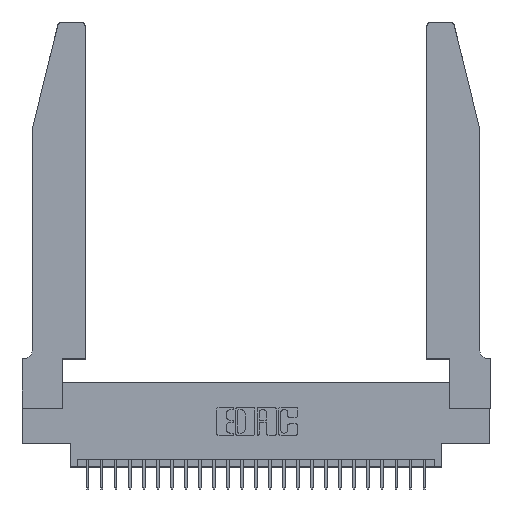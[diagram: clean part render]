
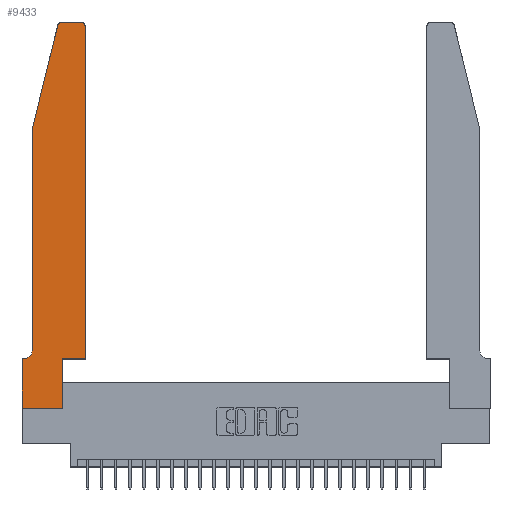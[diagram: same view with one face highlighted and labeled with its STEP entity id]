
A CAD part, top view. The second image highlights one B-rep face of the part: STEP entity #9433.
In plain terms, the highlighted planar face has unit normal (0, 0, 1).
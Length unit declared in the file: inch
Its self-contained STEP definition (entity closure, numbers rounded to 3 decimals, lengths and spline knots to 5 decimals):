
#201 = DIRECTION ( 'NONE',  ( 0., 0., 1. ) ) ;
#255 = CARTESIAN_POINT ( 'NONE',  ( 0.25487, 2.72718, 0.37 ) ) ;
#428 = EDGE_CURVE ( 'NONE', #19075, #12175, #15630, .T. ) ;
#579 = AXIS2_PLACEMENT_3D ( 'NONE', #21313, #201, #15273 ) ;
#582 = CARTESIAN_POINT ( 'NONE',  ( 0.4505, 0.35, 0.37 ) ) ;
#599 = DIRECTION ( 'NONE',  ( 0., -1., 0. ) ) ;
#766 = VERTEX_POINT ( 'NONE', #12396 ) ;
#1272 = CARTESIAN_POINT ( 'NONE',  ( 0.2865, 0.35, 0.37 ) ) ;
#1925 = VECTOR ( 'NONE', #23389, 39.37008 ) ;
#2009 = VERTEX_POINT ( 'NONE', #18621 ) ;
#2076 = VERTEX_POINT ( 'NONE', #255 ) ;
#2501 = VECTOR ( 'NONE', #21606, 39.37008 ) ;
#2733 = DIRECTION ( 'NONE',  ( -1., 0., 0. ) ) ;
#2997 = FACE_OUTER_BOUND ( 'NONE', #4580, .T. ) ;
#3164 = LINE ( 'NONE', #19623, #16791 ) ;
#3190 = CARTESIAN_POINT ( 'NONE',  ( 0.4505, 0.35, 0.37 ) ) ;
#3637 = DIRECTION ( 'NONE',  ( 1., 0., 0. ) ) ;
#3979 = ORIENTED_EDGE ( 'NONE', *, *, #20023, .T. ) ;
#4580 = EDGE_LOOP ( 'NONE', ( #16132, #8854, #22456, #3979, #19165, #18910, #22630, #10959, #16016, #23690, #14038, #8285 ) ) ;
#4980 = CARTESIAN_POINT ( 'NONE',  ( 0.0055, 0.42, 0.37 ) ) ;
#5750 = CARTESIAN_POINT ( 'NONE',  ( 0., 0.35, 0.37 ) ) ;
#5932 = CARTESIAN_POINT ( 'NONE',  ( 0.0755, 2., 0.37 ) ) ;
#6069 = LINE ( 'NONE', #582, #2501 ) ;
#7103 = CIRCLE ( 'NONE', #16468, 0.07 ) ;
#7587 = CARTESIAN_POINT ( 'NONE',  ( 0.4505, 2.72, 0.37 ) ) ;
#7709 = VECTOR ( 'NONE', #3637, 39.37008 ) ;
#7815 = VERTEX_POINT ( 'NONE', #7587 ) ;
#7955 = CARTESIAN_POINT ( 'NONE',  ( 0.2865, 0.35, 0.37 ) ) ;
#8285 = ORIENTED_EDGE ( 'NONE', *, *, #20357, .T. ) ;
#8297 = EDGE_CURVE ( 'NONE', #24174, #2009, #24781, .T. ) ;
#8361 = CARTESIAN_POINT ( 'NONE',  ( 0., 0., 0.37 ) ) ;
#8854 = ORIENTED_EDGE ( 'NONE', *, *, #17176, .T. ) ;
#9367 = LINE ( 'NONE', #20008, #7709 ) ;
#9433 = ADVANCED_FACE ( 'NONE', ( #2997 ), #18389, .T. ) ;
#9631 = CIRCLE ( 'NONE', #579, 0.03 ) ;
#10236 = CARTESIAN_POINT ( 'NONE',  ( 0.0755, 0.35, 0.37 ) ) ;
#10495 = CARTESIAN_POINT ( 'NONE',  ( 0.0055, 0.35, 0.37 ) ) ;
#10843 = EDGE_CURVE ( 'NONE', #15918, #26192, #7103, .T. ) ;
#10959 = ORIENTED_EDGE ( 'NONE', *, *, #19573, .T. ) ;
#11268 = DIRECTION ( 'NONE',  ( -1., 0., 0. ) ) ;
#11273 = EDGE_CURVE ( 'NONE', #26192, #24174, #24287, .T. ) ;
#11749 = VECTOR ( 'NONE', #21654, 39.37008 ) ;
#12175 = VERTEX_POINT ( 'NONE', #7955 ) ;
#12194 = LINE ( 'NONE', #5932, #21208 ) ;
#12396 = CARTESIAN_POINT ( 'NONE',  ( 0.0755, 2., 0.37 ) ) ;
#12456 = AXIS2_PLACEMENT_3D ( 'NONE', #5750, #15930, #24153 ) ;
#12502 = CARTESIAN_POINT ( 'NONE',  ( 0.284, 2.72, 0.37 ) ) ;
#13278 = CARTESIAN_POINT ( 'NONE',  ( 0.2605, 2.75, 0.37 ) ) ;
#13527 = CARTESIAN_POINT ( 'NONE',  ( 0.0755, 0.42, 0.37 ) ) ;
#14038 = ORIENTED_EDGE ( 'NONE', *, *, #14131, .T. ) ;
#14131 = EDGE_CURVE ( 'NONE', #22532, #7815, #17424, .T. ) ;
#15023 = EDGE_CURVE ( 'NONE', #2076, #766, #12194, .T. ) ;
#15273 = DIRECTION ( 'NONE',  ( 1., 0., 0. ) ) ;
#15482 = DIRECTION ( 'NONE',  ( 0., -1., 0. ) ) ;
#15630 = LINE ( 'NONE', #1272, #11749 ) ;
#15867 = CARTESIAN_POINT ( 'NONE',  ( 0.4505, 0.35, 0.37 ) ) ;
#15918 = VERTEX_POINT ( 'NONE', #13527 ) ;
#15930 = DIRECTION ( 'NONE',  ( 0., 0., 1. ) ) ;
#16016 = ORIENTED_EDGE ( 'NONE', *, *, #428, .T. ) ;
#16132 = ORIENTED_EDGE ( 'NONE', *, *, #16196, .T. ) ;
#16196 = EDGE_CURVE ( 'NONE', #20929, #24778, #23768, .T. ) ;
#16468 = AXIS2_PLACEMENT_3D ( 'NONE', #4980, #21458, #11268 ) ;
#16698 = VECTOR ( 'NONE', #599, 39.37008 ) ;
#16791 = VECTOR ( 'NONE', #15482, 39.37008 ) ;
#16854 = DIRECTION ( 'NONE',  ( 1., 0., 0. ) ) ;
#17142 = CARTESIAN_POINT ( 'NONE',  ( 0.284, 2.75, 0.37 ) ) ;
#17176 = EDGE_CURVE ( 'NONE', #24778, #2076, #20136, .T. ) ;
#17424 = LINE ( 'NONE', #15867, #24508 ) ;
#18389 = PLANE ( 'NONE',  #12456 ) ;
#18585 = CARTESIAN_POINT ( 'NONE',  ( 0.2865, 0., 0.37 ) ) ;
#18621 = CARTESIAN_POINT ( 'NONE',  ( 0., 0., 0.37 ) ) ;
#18910 = ORIENTED_EDGE ( 'NONE', *, *, #11273, .T. ) ;
#19075 = VERTEX_POINT ( 'NONE', #18585 ) ;
#19165 = ORIENTED_EDGE ( 'NONE', *, *, #10843, .T. ) ;
#19235 = VECTOR ( 'NONE', #2733, 39.37008 ) ;
#19573 = EDGE_CURVE ( 'NONE', #2009, #19075, #9367, .T. ) ;
#19623 = CARTESIAN_POINT ( 'NONE',  ( 0.0755, 2., 0.37 ) ) ;
#19924 = EDGE_CURVE ( 'NONE', #12175, #22532, #6069, .T. ) ;
#20008 = CARTESIAN_POINT ( 'NONE',  ( 0., 0., 0.37 ) ) ;
#20023 = EDGE_CURVE ( 'NONE', #766, #15918, #3164, .T. ) ;
#20136 = CIRCLE ( 'NONE', #20520, 0.03 ) ;
#20357 = EDGE_CURVE ( 'NONE', #7815, #20929, #9631, .T. ) ;
#20510 = DIRECTION ( 'NONE',  ( -0.239, -0.971, 0. ) ) ;
#20520 = AXIS2_PLACEMENT_3D ( 'NONE', #12502, #22705, #16854 ) ;
#20929 = VERTEX_POINT ( 'NONE', #23376 ) ;
#20945 = CARTESIAN_POINT ( 'NONE',  ( 0., 0.35, 0.37 ) ) ;
#21208 = VECTOR ( 'NONE', #20510, 39.37008 ) ;
#21313 = CARTESIAN_POINT ( 'NONE',  ( 0.4205, 2.72, 0.37 ) ) ;
#21458 = DIRECTION ( 'NONE',  ( 0., 0., -1. ) ) ;
#21606 = DIRECTION ( 'NONE',  ( 1., 0., 0. ) ) ;
#21654 = DIRECTION ( 'NONE',  ( 0., 1., 0. ) ) ;
#22456 = ORIENTED_EDGE ( 'NONE', *, *, #15023, .T. ) ;
#22532 = VERTEX_POINT ( 'NONE', #3190 ) ;
#22630 = ORIENTED_EDGE ( 'NONE', *, *, #8297, .T. ) ;
#22705 = DIRECTION ( 'NONE',  ( 0., 0., 1. ) ) ;
#23376 = CARTESIAN_POINT ( 'NONE',  ( 0.4205, 2.75, 0.37 ) ) ;
#23389 = DIRECTION ( 'NONE',  ( -1., 0., 0. ) ) ;
#23690 = ORIENTED_EDGE ( 'NONE', *, *, #19924, .T. ) ;
#23768 = LINE ( 'NONE', #13278, #19235 ) ;
#24153 = DIRECTION ( 'NONE',  ( 1., 0., 0. ) ) ;
#24174 = VERTEX_POINT ( 'NONE', #20945 ) ;
#24272 = DIRECTION ( 'NONE',  ( 0., 1., 0. ) ) ;
#24287 = LINE ( 'NONE', #10236, #1925 ) ;
#24508 = VECTOR ( 'NONE', #24272, 39.37008 ) ;
#24778 = VERTEX_POINT ( 'NONE', #17142 ) ;
#24781 = LINE ( 'NONE', #8361, #16698 ) ;
#26192 = VERTEX_POINT ( 'NONE', #10495 ) ;
